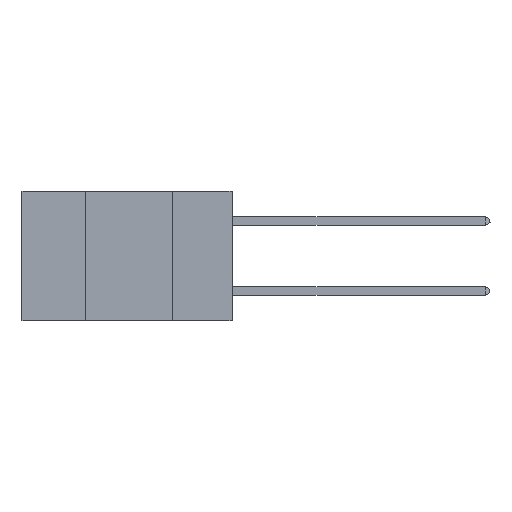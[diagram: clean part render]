
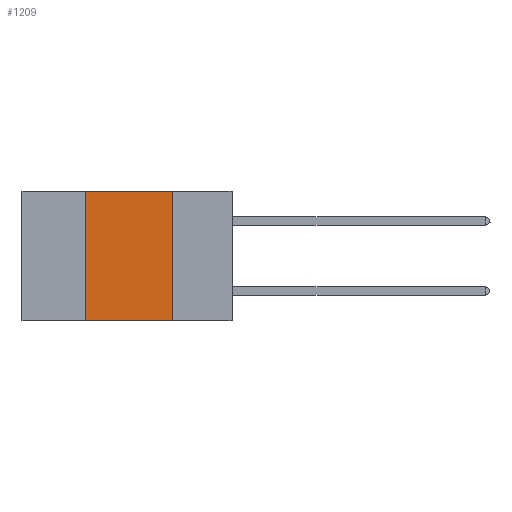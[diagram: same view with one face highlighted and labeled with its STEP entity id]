
A CAD part, left-side view. The second image highlights one B-rep face of the part: STEP entity #1209.
In plain terms, the highlighted planar face has unit normal (-1, 0, 0).
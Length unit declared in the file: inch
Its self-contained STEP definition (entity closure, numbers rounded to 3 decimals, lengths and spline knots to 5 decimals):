
#298 = EDGE_CURVE ( 'NONE', #17272, #19317, #2474, .T. ) ;
#514 = DIRECTION ( 'NONE',  ( 0., 0., -1. ) ) ;
#709 = LINE ( 'NONE', #11857, #18167 ) ;
#1209 = ADVANCED_FACE ( 'NONE', ( #10219 ), #10323, .F. ) ;
#2474 = LINE ( 'NONE', #5691, #13399 ) ;
#3245 = CARTESIAN_POINT ( 'NONE',  ( 0., 0.6, -0.37 ) ) ;
#3458 = LINE ( 'NONE', #3245, #8130 ) ;
#3669 = CARTESIAN_POINT ( 'NONE',  ( 0., 0.17, -0.37 ) ) ;
#4320 = EDGE_CURVE ( 'NONE', #19317, #14195, #709, .T. ) ;
#5139 = DIRECTION ( 'NONE',  ( 1., 0., 0. ) ) ;
#5691 = CARTESIAN_POINT ( 'NONE',  ( 0., 0.42, 0. ) ) ;
#7011 = CARTESIAN_POINT ( 'NONE',  ( 0., 0.6, 0. ) ) ;
#7595 = ORIENTED_EDGE ( 'NONE', *, *, #20429, .F. ) ;
#8130 = VECTOR ( 'NONE', #12917, 39.37008 ) ;
#8209 = AXIS2_PLACEMENT_3D ( 'NONE', #7011, #5139, #19672 ) ;
#8686 = CARTESIAN_POINT ( 'NONE',  ( 0., 0.17, 0. ) ) ;
#9988 = LINE ( 'NONE', #16310, #13895 ) ;
#10219 = FACE_OUTER_BOUND ( 'NONE', #15576, .T. ) ;
#10273 = ORIENTED_EDGE ( 'NONE', *, *, #16277, .T. ) ;
#10323 = PLANE ( 'NONE',  #8209 ) ;
#11857 = CARTESIAN_POINT ( 'NONE',  ( 0., 0.6, 0. ) ) ;
#12917 = DIRECTION ( 'NONE',  ( 0., -1., 0. ) ) ;
#13389 = DIRECTION ( 'NONE',  ( 0., -1., 0. ) ) ;
#13399 = VECTOR ( 'NONE', #16595, 39.37008 ) ;
#13450 = CARTESIAN_POINT ( 'NONE',  ( 0., 0.42, -0.37 ) ) ;
#13593 = CARTESIAN_POINT ( 'NONE',  ( 0., 0.42, 0. ) ) ;
#13895 = VECTOR ( 'NONE', #514, 39.37008 ) ;
#14195 = VERTEX_POINT ( 'NONE', #8686 ) ;
#15576 = EDGE_LOOP ( 'NONE', ( #7595, #19767, #17226, #10273 ) ) ;
#16277 = EDGE_CURVE ( 'NONE', #17272, #18577, #3458, .T. ) ;
#16310 = CARTESIAN_POINT ( 'NONE',  ( 0., 0.17, 0. ) ) ;
#16595 = DIRECTION ( 'NONE',  ( 0., 0., 1. ) ) ;
#17226 = ORIENTED_EDGE ( 'NONE', *, *, #298, .F. ) ;
#17272 = VERTEX_POINT ( 'NONE', #13450 ) ;
#18167 = VECTOR ( 'NONE', #13389, 39.37008 ) ;
#18577 = VERTEX_POINT ( 'NONE', #3669 ) ;
#19317 = VERTEX_POINT ( 'NONE', #13593 ) ;
#19672 = DIRECTION ( 'NONE',  ( 0., 0., -1. ) ) ;
#19767 = ORIENTED_EDGE ( 'NONE', *, *, #4320, .F. ) ;
#20429 = EDGE_CURVE ( 'NONE', #14195, #18577, #9988, .T. ) ;
